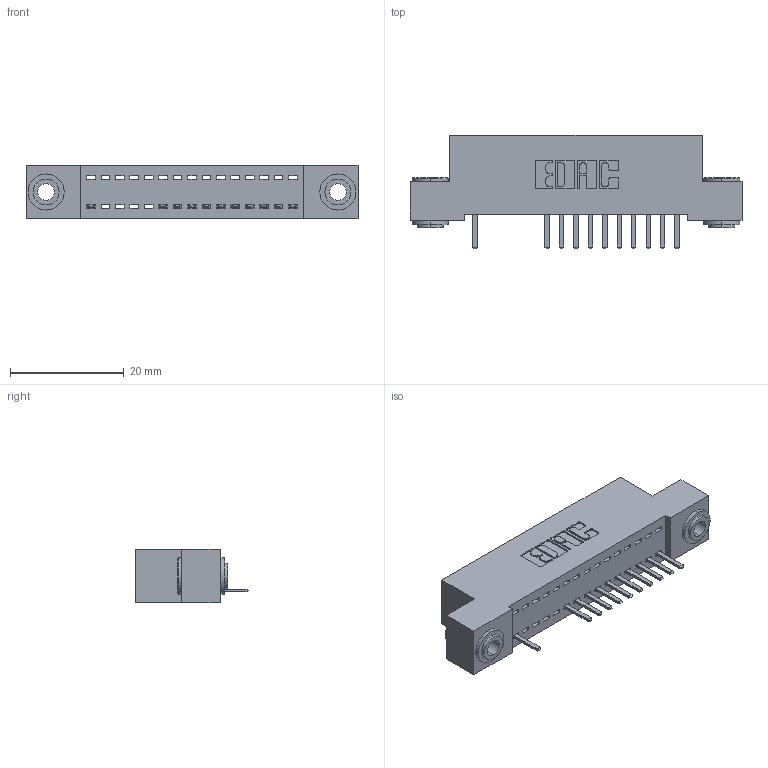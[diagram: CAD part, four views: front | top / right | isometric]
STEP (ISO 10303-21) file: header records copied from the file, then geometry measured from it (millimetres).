
FILE_DESCRIPTION (( 'STEP AP203' ), '1' );
FILE_NAME ('392-015-520-103.STEP', '2018-08-15T00:42:39', ( '' ), ( '' ), 'SwSTEP 2.0', 'SolidWorks 2016', '' );
FILE_SCHEMA (( 'CONFIG_CONTROL_DESIGN' ));
Length unit declared in the file: inch
Products named in the file (4): 342 Part_.156 TH; 345-292-001_345-293-120; 342-250-002_345-250-002-102; 392-015-520-103
Assembly tree (14 placements, depth 2):
  392-015-520-103
    342 Part_.156 TH
    345-292-001_345-293-120  x11
    342-250-002_345-250-002-102  x2
Bounding box: 58.42 x 20.02 x 9.4 mm (x, y, z)
Volume: 4968.3 mm3; surface area: 6679.4 mm2
Topology: 14 solids, 14 shells, 878 faces, 2567 edges, 1678 vertices
Faces by surface type: plane 608, cylinder 262, cone 8
Entity records: 13166 total; most frequent: CARTESIAN_POINT 2282, ORIENTED_EDGE 2218, DIRECTION 1997, EDGE_CURVE 1109, LINE 953, VECTOR 953, VERTEX_POINT 734, AXIS2_PLACEMENT_3D 522
